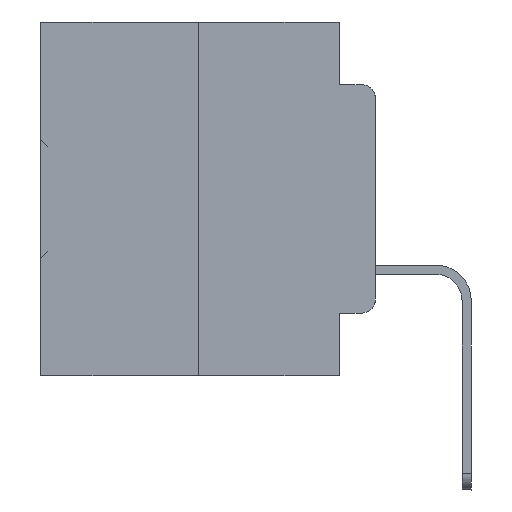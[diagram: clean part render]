
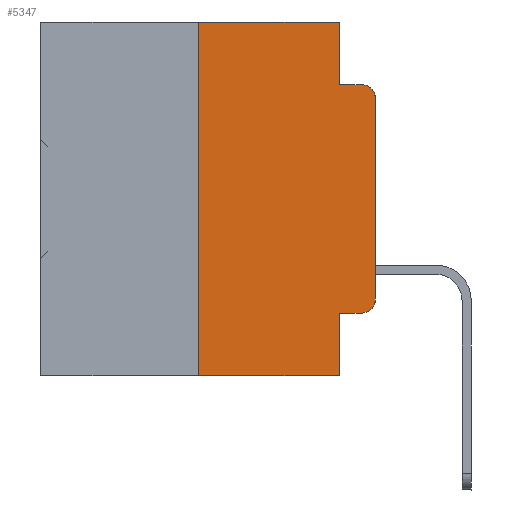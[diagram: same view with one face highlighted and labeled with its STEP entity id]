
A CAD part, left-side view. The second image highlights one B-rep face of the part: STEP entity #5347.
In plain terms, the highlighted planar face has unit normal (-1, 0, 0).
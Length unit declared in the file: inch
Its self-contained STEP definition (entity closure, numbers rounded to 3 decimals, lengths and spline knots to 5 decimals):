
#774 = VERTEX_POINT ( 'NONE', #17136 ) ;
#1977 = CARTESIAN_POINT ( 'NONE',  ( 0., 0.051, -0.4115 ) ) ;
#2184 = CARTESIAN_POINT ( 'NONE',  ( 0., 0.02, -0.1085 ) ) ;
#2203 = LINE ( 'NONE', #16354, #34596 ) ;
#2748 = EDGE_CURVE ( 'NONE', #22916, #20078, #36078, .T. ) ;
#2982 = VECTOR ( 'NONE', #37267, 39.37008 ) ;
#3233 = CARTESIAN_POINT ( 'NONE',  ( 0., 0.473, 0. ) ) ;
#4465 = CARTESIAN_POINT ( 'NONE',  ( 0., 0.02, -0.0885 ) ) ;
#4944 = EDGE_CURVE ( 'NONE', #10972, #24844, #2203, .T. ) ;
#5347 = ADVANCED_FACE ( 'NONE', ( #19786 ), #20067, .F. ) ;
#5693 = CARTESIAN_POINT ( 'NONE',  ( 0., 0.473, -0.5 ) ) ;
#5708 = VECTOR ( 'NONE', #11891, 39.37008 ) ;
#5870 = DIRECTION ( 'NONE',  ( 0., 0., 1. ) ) ;
#6507 = CARTESIAN_POINT ( 'NONE',  ( 0., 0.02, -0.4115 ) ) ;
#6800 = DIRECTION ( 'NONE',  ( 0., -1., 0. ) ) ;
#6925 = CARTESIAN_POINT ( 'NONE',  ( 0., 0., -0.3915 ) ) ;
#7527 = EDGE_CURVE ( 'NONE', #34557, #17555, #29972, .T. ) ;
#7634 = LINE ( 'NONE', #32156, #21544 ) ;
#8390 = CARTESIAN_POINT ( 'NONE',  ( 0., 0.051, 0. ) ) ;
#8418 = DIRECTION ( 'NONE',  ( 0., 0., -1. ) ) ;
#8618 = DIRECTION ( 'NONE',  ( 0., -1., 0. ) ) ;
#8674 = CARTESIAN_POINT ( 'NONE',  ( 0., 0.473, 0. ) ) ;
#9031 = EDGE_CURVE ( 'NONE', #27154, #37227, #33075, .T. ) ;
#9609 = EDGE_CURVE ( 'NONE', #10972, #27154, #29390, .T. ) ;
#9746 = LINE ( 'NONE', #8390, #2982 ) ;
#10265 = CARTESIAN_POINT ( 'NONE',  ( 0., 0.02, -0.3915 ) ) ;
#10346 = AXIS2_PLACEMENT_3D ( 'NONE', #8674, #25451, #8418 ) ;
#10806 = ORIENTED_EDGE ( 'NONE', *, *, #9609, .T. ) ;
#10911 = VERTEX_POINT ( 'NONE', #28222 ) ;
#10972 = VERTEX_POINT ( 'NONE', #1977 ) ;
#10982 = VECTOR ( 'NONE', #6800, 39.37008 ) ;
#11355 = CARTESIAN_POINT ( 'NONE',  ( 0., 0.25, 0. ) ) ;
#11421 = LINE ( 'NONE', #5693, #29837 ) ;
#11519 = CARTESIAN_POINT ( 'NONE',  ( 0., 0.051, -0.5 ) ) ;
#11721 = DIRECTION ( 'NONE',  ( 0., -1., 0. ) ) ;
#11827 = LINE ( 'NONE', #11355, #12270 ) ;
#11891 = DIRECTION ( 'NONE',  ( 0., -1., 0. ) ) ;
#12270 = VECTOR ( 'NONE', #14359, 39.37008 ) ;
#14359 = DIRECTION ( 'NONE',  ( 0., 0., 1. ) ) ;
#15941 = ORIENTED_EDGE ( 'NONE', *, *, #29983, .F. ) ;
#16354 = CARTESIAN_POINT ( 'NONE',  ( 0., 0.051, 0. ) ) ;
#17136 = CARTESIAN_POINT ( 'NONE',  ( 0., 0.051, -0.0885 ) ) ;
#17555 = VERTEX_POINT ( 'NONE', #33432 ) ;
#19009 = DIRECTION ( 'NONE',  ( -1., 0., 0. ) ) ;
#19246 = DIRECTION ( 'NONE',  ( 0., 0., -1. ) ) ;
#19786 = FACE_OUTER_BOUND ( 'NONE', #36057, .T. ) ;
#20067 = PLANE ( 'NONE',  #10346 ) ;
#20078 = VERTEX_POINT ( 'NONE', #4465 ) ;
#20577 = EDGE_CURVE ( 'NONE', #37227, #22916, #7634, .T. ) ;
#20605 = CARTESIAN_POINT ( 'NONE',  ( 0., 0.25, 0. ) ) ;
#21096 = ORIENTED_EDGE ( 'NONE', *, *, #9031, .T. ) ;
#21516 = ORIENTED_EDGE ( 'NONE', *, *, #7527, .F. ) ;
#21544 = VECTOR ( 'NONE', #5870, 39.37008 ) ;
#21813 = ORIENTED_EDGE ( 'NONE', *, *, #25452, .F. ) ;
#22916 = VERTEX_POINT ( 'NONE', #23862 ) ;
#23695 = EDGE_CURVE ( 'NONE', #10911, #24844, #11421, .T. ) ;
#23862 = CARTESIAN_POINT ( 'NONE',  ( 0., 0., -0.1085 ) ) ;
#24005 = CARTESIAN_POINT ( 'NONE',  ( 0., 0.051, -0.4115 ) ) ;
#24844 = VERTEX_POINT ( 'NONE', #11519 ) ;
#25451 = DIRECTION ( 'NONE',  ( 1., 0., 0. ) ) ;
#25452 = EDGE_CURVE ( 'NONE', #10911, #34557, #11827, .T. ) ;
#26156 = ORIENTED_EDGE ( 'NONE', *, *, #2748, .T. ) ;
#26309 = ORIENTED_EDGE ( 'NONE', *, *, #4944, .F. ) ;
#26383 = EDGE_CURVE ( 'NONE', #774, #20078, #30179, .T. ) ;
#27154 = VERTEX_POINT ( 'NONE', #6507 ) ;
#27310 = DIRECTION ( 'NONE',  ( 0., 0., -1. ) ) ;
#27804 = DIRECTION ( 'NONE',  ( -1., 0., 0. ) ) ;
#28222 = CARTESIAN_POINT ( 'NONE',  ( 0., 0.25, -0.5 ) ) ;
#28359 = VECTOR ( 'NONE', #11721, 39.37008 ) ;
#28766 = ORIENTED_EDGE ( 'NONE', *, *, #20577, .T. ) ;
#28919 = CARTESIAN_POINT ( 'NONE',  ( 0., 0.051, -0.0885 ) ) ;
#29235 = AXIS2_PLACEMENT_3D ( 'NONE', #2184, #27804, #31496 ) ;
#29390 = LINE ( 'NONE', #24005, #10982 ) ;
#29837 = VECTOR ( 'NONE', #8618, 39.37008 ) ;
#29972 = LINE ( 'NONE', #3233, #5708 ) ;
#29983 = EDGE_CURVE ( 'NONE', #17555, #774, #9746, .T. ) ;
#30179 = LINE ( 'NONE', #28919, #28359 ) ;
#31496 = DIRECTION ( 'NONE',  ( 0., 0., -1. ) ) ;
#32156 = CARTESIAN_POINT ( 'NONE',  ( 0., 0., 0. ) ) ;
#33075 = CIRCLE ( 'NONE', #37106, 0.02 ) ;
#33432 = CARTESIAN_POINT ( 'NONE',  ( 0., 0.051, 0. ) ) ;
#34557 = VERTEX_POINT ( 'NONE', #20605 ) ;
#34596 = VECTOR ( 'NONE', #19246, 39.37008 ) ;
#34704 = ORIENTED_EDGE ( 'NONE', *, *, #23695, .T. ) ;
#36057 = EDGE_LOOP ( 'NONE', ( #28766, #26156, #37271, #15941, #21516, #21813, #34704, #26309, #10806, #21096 ) ) ;
#36078 = CIRCLE ( 'NONE', #29235, 0.02 ) ;
#37106 = AXIS2_PLACEMENT_3D ( 'NONE', #10265, #19009, #27310 ) ;
#37227 = VERTEX_POINT ( 'NONE', #6925 ) ;
#37267 = DIRECTION ( 'NONE',  ( 0., 0., -1. ) ) ;
#37271 = ORIENTED_EDGE ( 'NONE', *, *, #26383, .F. ) ;
